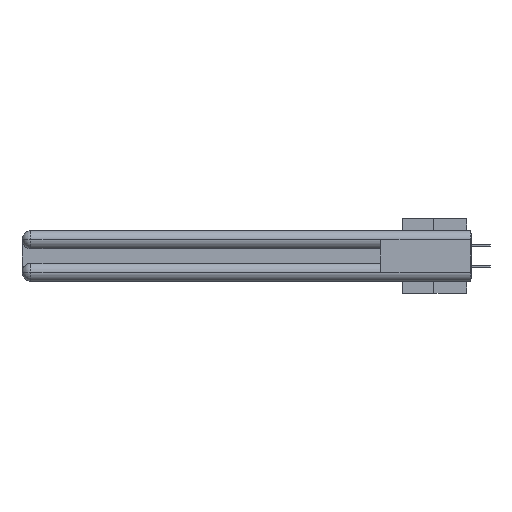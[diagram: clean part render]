
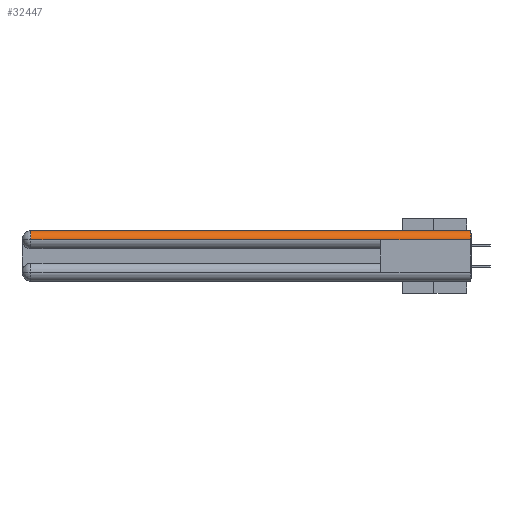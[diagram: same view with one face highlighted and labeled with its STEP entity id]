
A CAD part, left-side view. The second image highlights one B-rep face of the part: STEP entity #32447.
In plain terms, the highlighted cylindrical face has radius 1.562 mm (diameter 3.124 mm), a partial arc.
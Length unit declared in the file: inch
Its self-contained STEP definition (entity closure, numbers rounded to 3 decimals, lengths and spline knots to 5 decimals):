
#894 = CARTESIAN_POINT ( 'NONE',  ( 0.0615, 0., -0.0615 ) ) ;
#2970 = ORIENTED_EDGE ( 'NONE', *, *, #23077, .F. ) ;
#4249 = AXIS2_PLACEMENT_3D ( 'NONE', #894, #11920, #28331 ) ;
#4391 = ORIENTED_EDGE ( 'NONE', *, *, #9596, .F. ) ;
#5498 = ORIENTED_EDGE ( 'NONE', *, *, #20076, .F. ) ;
#5768 = FACE_OUTER_BOUND ( 'NONE', #15907, .T. ) ;
#7075 = DIRECTION ( 'NONE',  ( 0., 1., 0. ) ) ;
#7269 = CARTESIAN_POINT ( 'NONE',  ( 0.0615, 0., 0. ) ) ;
#7741 = CARTESIAN_POINT ( 'NONE',  ( 0., 2.94, -0.0615 ) ) ;
#7743 = CARTESIAN_POINT ( 'NONE',  ( 0., 0., -0.0615 ) ) ;
#7858 = CYLINDRICAL_SURFACE ( 'NONE', #16253, 0.0615 ) ;
#8530 = DIRECTION ( 'NONE',  ( 0., -1., 0. ) ) ;
#8732 = DIRECTION ( 'NONE',  ( 0., 0., 1. ) ) ;
#9596 = EDGE_CURVE ( 'NONE', #19989, #21909, #17926, .T. ) ;
#9631 = CARTESIAN_POINT ( 'NONE',  ( 0., 3., -0.0615 ) ) ;
#10291 = CARTESIAN_POINT ( 'NONE',  ( 0., 3., -0.0615 ) ) ;
#11710 = CARTESIAN_POINT ( 'NONE',  ( 0., 0.6, -0.0615 ) ) ;
#11920 = DIRECTION ( 'NONE',  ( 0., -1., 0. ) ) ;
#13414 = VECTOR ( 'NONE', #8530, 39.37008 ) ;
#14415 = DIRECTION ( 'NONE',  ( 0., 1., 0. ) ) ;
#14514 = VERTEX_POINT ( 'NONE', #7741 ) ;
#14657 = DIRECTION ( 'NONE',  ( 0., 0., 1. ) ) ;
#14999 = VECTOR ( 'NONE', #7075, 39.37008 ) ;
#15450 = AXIS2_PLACEMENT_3D ( 'NONE', #22731, #16897, #8732 ) ;
#15907 = EDGE_LOOP ( 'NONE', ( #5498, #24042, #26157, #2970, #4391 ) ) ;
#16253 = AXIS2_PLACEMENT_3D ( 'NONE', #25426, #14415, #14657 ) ;
#16897 = DIRECTION ( 'NONE',  ( 0., -1., 0. ) ) ;
#17926 = CIRCLE ( 'NONE', #4249, 0.0615 ) ;
#18542 = VERTEX_POINT ( 'NONE', #20159 ) ;
#18913 = CIRCLE ( 'NONE', #15450, 0.0615 ) ;
#19989 = VERTEX_POINT ( 'NONE', #7269 ) ;
#20076 = EDGE_CURVE ( 'NONE', #18542, #19989, #25145, .T. ) ;
#20159 = CARTESIAN_POINT ( 'NONE',  ( 0.0615, 2.94, 0. ) ) ;
#21654 = VERTEX_POINT ( 'NONE', #11710 ) ;
#21909 = VERTEX_POINT ( 'NONE', #7743 ) ;
#22731 = CARTESIAN_POINT ( 'NONE',  ( 0.0615, 2.94, -0.0615 ) ) ;
#23077 = EDGE_CURVE ( 'NONE', #21909, #21654, #33474, .T. ) ;
#23315 = EDGE_CURVE ( 'NONE', #18542, #14514, #18913, .T. ) ;
#24042 = ORIENTED_EDGE ( 'NONE', *, *, #23315, .T. ) ;
#25053 = CARTESIAN_POINT ( 'NONE',  ( 0.0615, 0., 0. ) ) ;
#25145 = LINE ( 'NONE', #25053, #13414 ) ;
#25426 = CARTESIAN_POINT ( 'NONE',  ( 0.0615, 0., -0.0615 ) ) ;
#26157 = ORIENTED_EDGE ( 'NONE', *, *, #29546, .T. ) ;
#27660 = VECTOR ( 'NONE', #32423, 39.37008 ) ;
#28331 = DIRECTION ( 'NONE',  ( 1., 0., 0. ) ) ;
#29546 = EDGE_CURVE ( 'NONE', #14514, #21654, #34912, .T. ) ;
#32423 = DIRECTION ( 'NONE',  ( 0., -1., 0. ) ) ;
#32447 = ADVANCED_FACE ( 'NONE', ( #5768 ), #7858, .T. ) ;
#33474 = LINE ( 'NONE', #9631, #14999 ) ;
#34912 = LINE ( 'NONE', #10291, #27660 ) ;
